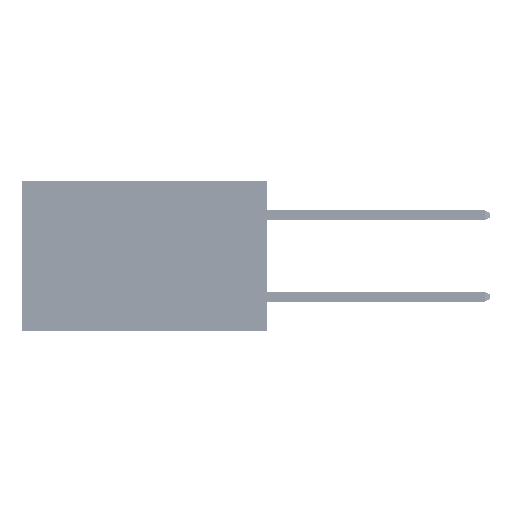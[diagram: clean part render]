
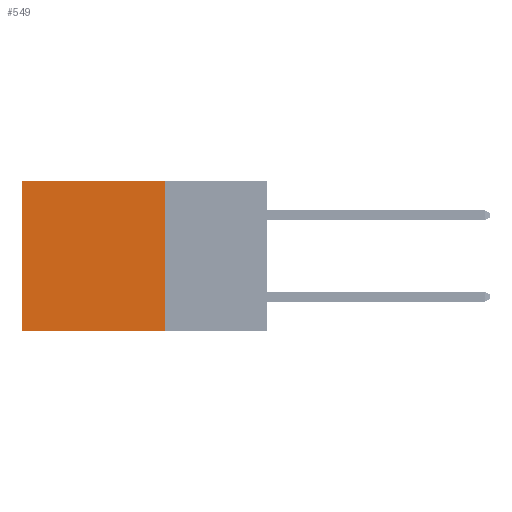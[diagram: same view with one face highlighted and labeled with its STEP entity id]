
A CAD part, left-side view. The second image highlights one B-rep face of the part: STEP entity #549.
In plain terms, the highlighted planar face has unit normal (-1, 0, 0).
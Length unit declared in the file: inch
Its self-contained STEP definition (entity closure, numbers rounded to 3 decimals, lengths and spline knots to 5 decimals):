
#549 = ADVANCED_FACE ( 'NONE', ( #34324 ), #49390, .F. ) ;
#5065 = VERTEX_POINT ( 'NONE', #16048 ) ;
#5991 = CARTESIAN_POINT ( 'NONE',  ( 0.2875, 0.6, -0.37 ) ) ;
#6317 = CARTESIAN_POINT ( 'NONE',  ( 0.2875, 0.6, 0. ) ) ;
#7121 = CARTESIAN_POINT ( 'NONE',  ( 0.2875, 0.25, -0.37 ) ) ;
#7235 = EDGE_LOOP ( 'NONE', ( #32128, #17659, #7891, #9256 ) ) ;
#7891 = ORIENTED_EDGE ( 'NONE', *, *, #31320, .F. ) ;
#8876 = CARTESIAN_POINT ( 'NONE',  ( 0.2875, 0.25, -0.37 ) ) ;
#9256 = ORIENTED_EDGE ( 'NONE', *, *, #13365, .T. ) ;
#13365 = EDGE_CURVE ( 'NONE', #5065, #31172, #41558, .T. ) ;
#14208 = VERTEX_POINT ( 'NONE', #5991 ) ;
#14417 = LINE ( 'NONE', #35133, #42440 ) ;
#15461 = AXIS2_PLACEMENT_3D ( 'NONE', #37318, #37810, #21667 ) ;
#16048 = CARTESIAN_POINT ( 'NONE',  ( 0.2875, 0.25, 0. ) ) ;
#17659 = ORIENTED_EDGE ( 'NONE', *, *, #21265, .F. ) ;
#20232 = DIRECTION ( 'NONE',  ( 0., 1., 0. ) ) ;
#21265 = EDGE_CURVE ( 'NONE', #38619, #14208, #49817, .T. ) ;
#21667 = DIRECTION ( 'NONE',  ( 0., 0., -1. ) ) ;
#22445 = CARTESIAN_POINT ( 'NONE',  ( 0.2875, 0.6, 0. ) ) ;
#24616 = VECTOR ( 'NONE', #30390, 39.37008 ) ;
#29112 = DIRECTION ( 'NONE',  ( 0., 1., 0. ) ) ;
#30390 = DIRECTION ( 'NONE',  ( 0., 0., -1. ) ) ;
#31172 = VERTEX_POINT ( 'NONE', #22445 ) ;
#31320 = EDGE_CURVE ( 'NONE', #5065, #38619, #14417, .T. ) ;
#32128 = ORIENTED_EDGE ( 'NONE', *, *, #37824, .T. ) ;
#34324 = FACE_OUTER_BOUND ( 'NONE', #7235, .T. ) ;
#35133 = CARTESIAN_POINT ( 'NONE',  ( 0.2875, 0.25, 0. ) ) ;
#37318 = CARTESIAN_POINT ( 'NONE',  ( 0.2875, 0.25, 0. ) ) ;
#37810 = DIRECTION ( 'NONE',  ( 1., 0., 0. ) ) ;
#37824 = EDGE_CURVE ( 'NONE', #31172, #14208, #38257, .T. ) ;
#38257 = LINE ( 'NONE', #6317, #24616 ) ;
#38619 = VERTEX_POINT ( 'NONE', #7121 ) ;
#41276 = CARTESIAN_POINT ( 'NONE',  ( 0.2875, 0.25, 0. ) ) ;
#41558 = LINE ( 'NONE', #41276, #42797 ) ;
#42440 = VECTOR ( 'NONE', #50715, 39.37008 ) ;
#42797 = VECTOR ( 'NONE', #29112, 39.37008 ) ;
#48557 = VECTOR ( 'NONE', #20232, 39.37008 ) ;
#49390 = PLANE ( 'NONE',  #15461 ) ;
#49817 = LINE ( 'NONE', #8876, #48557 ) ;
#50715 = DIRECTION ( 'NONE',  ( 0., 0., -1. ) ) ;
